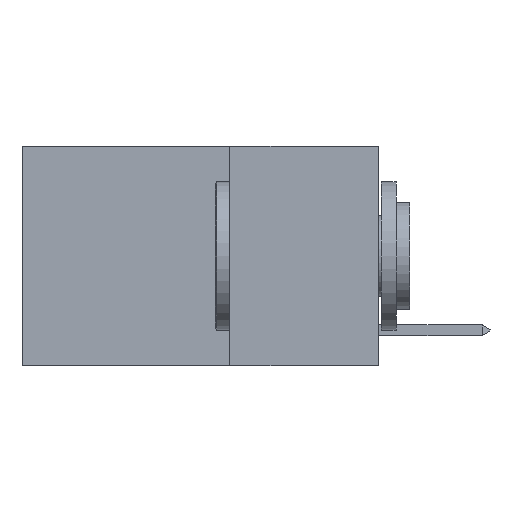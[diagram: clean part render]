
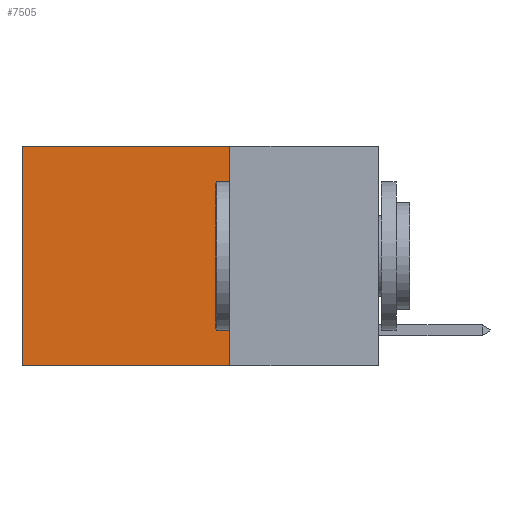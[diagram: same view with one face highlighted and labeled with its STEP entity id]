
A CAD part, left-side view. The second image highlights one B-rep face of the part: STEP entity #7505.
In plain terms, the highlighted planar face has unit normal (-1, 0, 0).
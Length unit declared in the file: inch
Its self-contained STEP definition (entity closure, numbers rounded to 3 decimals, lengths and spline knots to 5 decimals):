
#507 = LINE ( 'NONE', #6026, #11322 ) ;
#1577 = ORIENTED_EDGE ( 'NONE', *, *, #2446, .F. ) ;
#1929 = ORIENTED_EDGE ( 'NONE', *, *, #7777, .T. ) ;
#2434 = EDGE_CURVE ( 'NONE', #2936, #11716, #507, .T. ) ;
#2446 = EDGE_CURVE ( 'NONE', #10792, #5835, #9679, .T. ) ;
#2936 = VERTEX_POINT ( 'NONE', #7248 ) ;
#3096 = AXIS2_PLACEMENT_3D ( 'NONE', #7728, #6994, #7938 ) ;
#3142 = EDGE_CURVE ( 'NONE', #2936, #10792, #3739, .T. ) ;
#3739 = LINE ( 'NONE', #13035, #6104 ) ;
#4996 = DIRECTION ( 'NONE',  ( 0., 0., -1. ) ) ;
#5835 = VERTEX_POINT ( 'NONE', #13348 ) ;
#6026 = CARTESIAN_POINT ( 'NONE',  ( 0.2625, 0.25, 0. ) ) ;
#6104 = VECTOR ( 'NONE', #7524, 39.37008 ) ;
#6145 = EDGE_LOOP ( 'NONE', ( #1929, #1577, #8430, #10335 ) ) ;
#6473 = CARTESIAN_POINT ( 'NONE',  ( 0.2625, 0.6, 0. ) ) ;
#6564 = DIRECTION ( 'NONE',  ( 0., 1., 0. ) ) ;
#6994 = DIRECTION ( 'NONE',  ( 1., 0., 0. ) ) ;
#7248 = CARTESIAN_POINT ( 'NONE',  ( 0.2625, 0.25, 0. ) ) ;
#7505 = ADVANCED_FACE ( 'NONE', ( #13787 ), #9102, .F. ) ;
#7524 = DIRECTION ( 'NONE',  ( 0., 0., -1. ) ) ;
#7728 = CARTESIAN_POINT ( 'NONE',  ( 0.2625, 0.25, 0. ) ) ;
#7777 = EDGE_CURVE ( 'NONE', #11716, #5835, #10083, .T. ) ;
#7938 = DIRECTION ( 'NONE',  ( 0., 0., -1. ) ) ;
#7946 = CARTESIAN_POINT ( 'NONE',  ( 0.2625, 0.25, -0.37 ) ) ;
#8430 = ORIENTED_EDGE ( 'NONE', *, *, #3142, .F. ) ;
#8455 = CARTESIAN_POINT ( 'NONE',  ( 0.2625, 0.6, 0. ) ) ;
#8864 = DIRECTION ( 'NONE',  ( 0., 1., 0. ) ) ;
#9102 = PLANE ( 'NONE',  #3096 ) ;
#9679 = LINE ( 'NONE', #7946, #13344 ) ;
#10083 = LINE ( 'NONE', #8455, #11581 ) ;
#10335 = ORIENTED_EDGE ( 'NONE', *, *, #2434, .T. ) ;
#10792 = VERTEX_POINT ( 'NONE', #14459 ) ;
#11322 = VECTOR ( 'NONE', #6564, 39.37008 ) ;
#11581 = VECTOR ( 'NONE', #4996, 39.37008 ) ;
#11716 = VERTEX_POINT ( 'NONE', #6473 ) ;
#13035 = CARTESIAN_POINT ( 'NONE',  ( 0.2625, 0.25, 0. ) ) ;
#13344 = VECTOR ( 'NONE', #8864, 39.37008 ) ;
#13348 = CARTESIAN_POINT ( 'NONE',  ( 0.2625, 0.6, -0.37 ) ) ;
#13787 = FACE_OUTER_BOUND ( 'NONE', #6145, .T. ) ;
#14459 = CARTESIAN_POINT ( 'NONE',  ( 0.2625, 0.25, -0.37 ) ) ;
